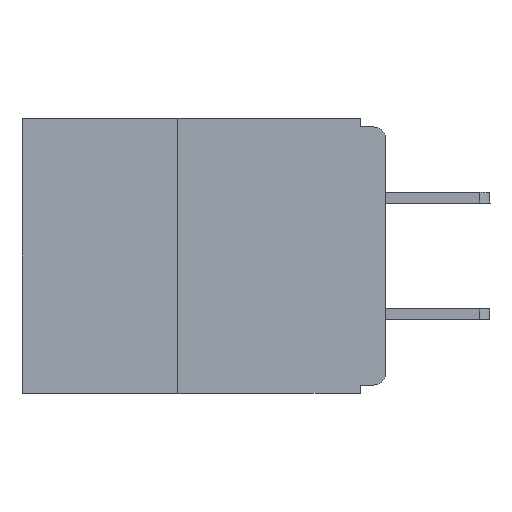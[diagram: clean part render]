
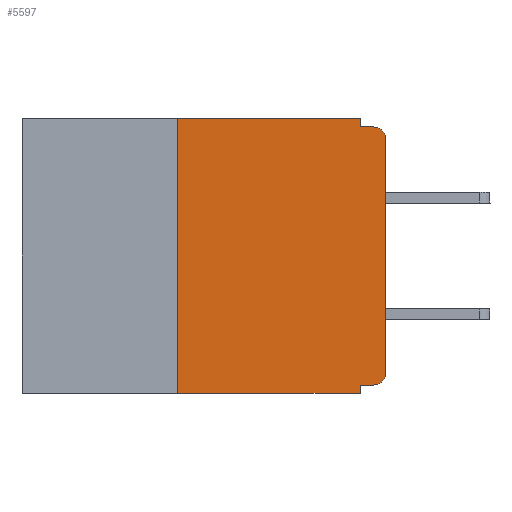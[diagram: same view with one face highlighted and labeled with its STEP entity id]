
A CAD part, left-side view. The second image highlights one B-rep face of the part: STEP entity #5597.
In plain terms, the highlighted planar face has unit normal (-1, 0, 0).
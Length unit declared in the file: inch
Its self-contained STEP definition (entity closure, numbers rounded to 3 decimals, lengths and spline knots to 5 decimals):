
#288 = CARTESIAN_POINT ( 'NONE',  ( 0., 0.015, -0.025 ) ) ;
#307 = CARTESIAN_POINT ( 'NONE',  ( 0., 0.015, -0.01 ) ) ;
#333 = DIRECTION ( 'NONE',  ( 0., 0., -1. ) ) ;
#477 = VECTOR ( 'NONE', #9121, 39.37008 ) ;
#650 = DIRECTION ( 'NONE',  ( 1., 0., 0. ) ) ;
#723 = VERTEX_POINT ( 'NONE', #7053 ) ;
#757 = CARTESIAN_POINT ( 'NONE',  ( 0., 0., -0.025 ) ) ;
#867 = ORIENTED_EDGE ( 'NONE', *, *, #4224, .F. ) ;
#1179 = DIRECTION ( 'NONE',  ( -1., 0., 0. ) ) ;
#1321 = VERTEX_POINT ( 'NONE', #5589 ) ;
#1565 = DIRECTION ( 'NONE',  ( 0., 0., -1. ) ) ;
#1728 = EDGE_LOOP ( 'NONE', ( #3768, #7342, #10377, #3603, #867, #6551, #11092, #7925, #9289, #9010 ) ) ;
#1787 = DIRECTION ( 'NONE',  ( 0., 1., 0. ) ) ;
#2169 = CIRCLE ( 'NONE', #2929, 0.015 ) ;
#2313 = EDGE_CURVE ( 'NONE', #5145, #11129, #7800, .T. ) ;
#2382 = LINE ( 'NONE', #4875, #3338 ) ;
#2719 = VECTOR ( 'NONE', #1787, 39.37008 ) ;
#2871 = VECTOR ( 'NONE', #7517, 39.37008 ) ;
#2929 = AXIS2_PLACEMENT_3D ( 'NONE', #288, #1179, #8337 ) ;
#3002 = DIRECTION ( 'NONE',  ( 0., 0., -1. ) ) ;
#3338 = VECTOR ( 'NONE', #6630, 39.37008 ) ;
#3349 = PLANE ( 'NONE',  #10792 ) ;
#3438 = EDGE_CURVE ( 'NONE', #3942, #7280, #6915, .T. ) ;
#3603 = ORIENTED_EDGE ( 'NONE', *, *, #2313, .F. ) ;
#3768 = ORIENTED_EDGE ( 'NONE', *, *, #3438, .T. ) ;
#3942 = VERTEX_POINT ( 'NONE', #10055 ) ;
#4000 = CARTESIAN_POINT ( 'NONE',  ( 0., 0.031, -0.33 ) ) ;
#4100 = FACE_OUTER_BOUND ( 'NONE', #1728, .T. ) ;
#4166 = CARTESIAN_POINT ( 'NONE',  ( 0., 0., -0.01 ) ) ;
#4206 = DIRECTION ( 'NONE',  ( 0., -1., 0. ) ) ;
#4224 = EDGE_CURVE ( 'NONE', #7465, #5145, #4528, .T. ) ;
#4262 = VECTOR ( 'NONE', #4633, 39.37008 ) ;
#4411 = LINE ( 'NONE', #6773, #2871 ) ;
#4425 = CARTESIAN_POINT ( 'NONE',  ( 0., 0., -0.32 ) ) ;
#4528 = LINE ( 'NONE', #9770, #4262 ) ;
#4536 = EDGE_CURVE ( 'NONE', #11129, #5330, #7982, .T. ) ;
#4633 = DIRECTION ( 'NONE',  ( 0., -1., 0. ) ) ;
#4646 = CARTESIAN_POINT ( 'NONE',  ( 0., 0.031, 0. ) ) ;
#4875 = CARTESIAN_POINT ( 'NONE',  ( 0., 0.437, -0.33 ) ) ;
#5145 = VERTEX_POINT ( 'NONE', #4646 ) ;
#5330 = VERTEX_POINT ( 'NONE', #307 ) ;
#5566 = CIRCLE ( 'NONE', #6792, 0.015 ) ;
#5589 = CARTESIAN_POINT ( 'NONE',  ( 0., 0.25, -0.33 ) ) ;
#5597 = ADVANCED_FACE ( 'NONE', ( #4100 ), #3349, .F. ) ;
#5756 = EDGE_CURVE ( 'NONE', #7501, #723, #8497, .T. ) ;
#5837 = LINE ( 'NONE', #10748, #6098 ) ;
#5983 = EDGE_CURVE ( 'NONE', #7280, #5330, #2169, .T. ) ;
#6098 = VECTOR ( 'NONE', #3002, 39.37008 ) ;
#6551 = ORIENTED_EDGE ( 'NONE', *, *, #8998, .F. ) ;
#6630 = DIRECTION ( 'NONE',  ( 0., -1., 0. ) ) ;
#6638 = CARTESIAN_POINT ( 'NONE',  ( 0., 0.015, -0.32 ) ) ;
#6773 = CARTESIAN_POINT ( 'NONE',  ( 0., 0.25, -0.33 ) ) ;
#6792 = AXIS2_PLACEMENT_3D ( 'NONE', #9052, #8117, #333 ) ;
#6915 = LINE ( 'NONE', #11229, #9892 ) ;
#7053 = CARTESIAN_POINT ( 'NONE',  ( 0., 0.031, -0.32 ) ) ;
#7280 = VERTEX_POINT ( 'NONE', #757 ) ;
#7299 = CARTESIAN_POINT ( 'NONE',  ( 0., 0.031, 0. ) ) ;
#7339 = EDGE_CURVE ( 'NONE', #723, #7446, #5837, .T. ) ;
#7342 = ORIENTED_EDGE ( 'NONE', *, *, #5983, .T. ) ;
#7446 = VERTEX_POINT ( 'NONE', #4000 ) ;
#7456 = CARTESIAN_POINT ( 'NONE',  ( 0., 0.25, 0. ) ) ;
#7465 = VERTEX_POINT ( 'NONE', #7456 ) ;
#7501 = VERTEX_POINT ( 'NONE', #6638 ) ;
#7517 = DIRECTION ( 'NONE',  ( 0., 0., 1. ) ) ;
#7800 = LINE ( 'NONE', #7299, #477 ) ;
#7925 = ORIENTED_EDGE ( 'NONE', *, *, #7339, .F. ) ;
#7982 = LINE ( 'NONE', #4166, #8647 ) ;
#8117 = DIRECTION ( 'NONE',  ( -1., 0., 0. ) ) ;
#8337 = DIRECTION ( 'NONE',  ( 0., 0., -1. ) ) ;
#8497 = LINE ( 'NONE', #4425, #2719 ) ;
#8553 = CARTESIAN_POINT ( 'NONE',  ( 0., 0.437, 0. ) ) ;
#8647 = VECTOR ( 'NONE', #4206, 39.37008 ) ;
#8664 = DIRECTION ( 'NONE',  ( 0., 0., 1. ) ) ;
#8740 = CARTESIAN_POINT ( 'NONE',  ( 0., 0.031, -0.01 ) ) ;
#8998 = EDGE_CURVE ( 'NONE', #1321, #7465, #4411, .T. ) ;
#9010 = ORIENTED_EDGE ( 'NONE', *, *, #9757, .T. ) ;
#9052 = CARTESIAN_POINT ( 'NONE',  ( 0., 0.015, -0.305 ) ) ;
#9121 = DIRECTION ( 'NONE',  ( 0., 0., -1. ) ) ;
#9289 = ORIENTED_EDGE ( 'NONE', *, *, #5756, .F. ) ;
#9757 = EDGE_CURVE ( 'NONE', #7501, #3942, #5566, .T. ) ;
#9770 = CARTESIAN_POINT ( 'NONE',  ( 0., 0.437, 0. ) ) ;
#9892 = VECTOR ( 'NONE', #8664, 39.37008 ) ;
#10055 = CARTESIAN_POINT ( 'NONE',  ( 0., 0., -0.305 ) ) ;
#10377 = ORIENTED_EDGE ( 'NONE', *, *, #4536, .F. ) ;
#10748 = CARTESIAN_POINT ( 'NONE',  ( 0., 0.031, -0.33 ) ) ;
#10792 = AXIS2_PLACEMENT_3D ( 'NONE', #8553, #650, #1565 ) ;
#10904 = EDGE_CURVE ( 'NONE', #1321, #7446, #2382, .T. ) ;
#11092 = ORIENTED_EDGE ( 'NONE', *, *, #10904, .T. ) ;
#11129 = VERTEX_POINT ( 'NONE', #8740 ) ;
#11229 = CARTESIAN_POINT ( 'NONE',  ( 0., 0., 0. ) ) ;
